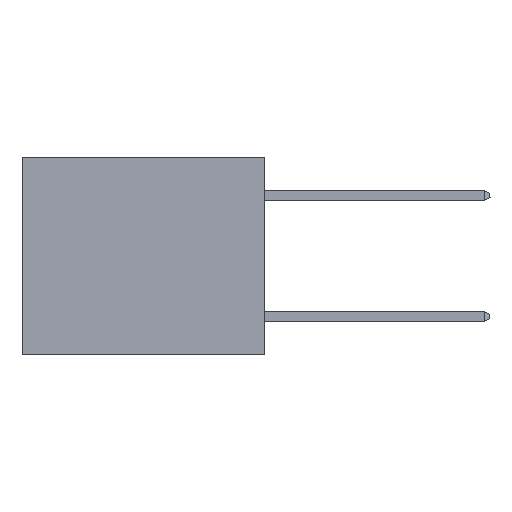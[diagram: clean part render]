
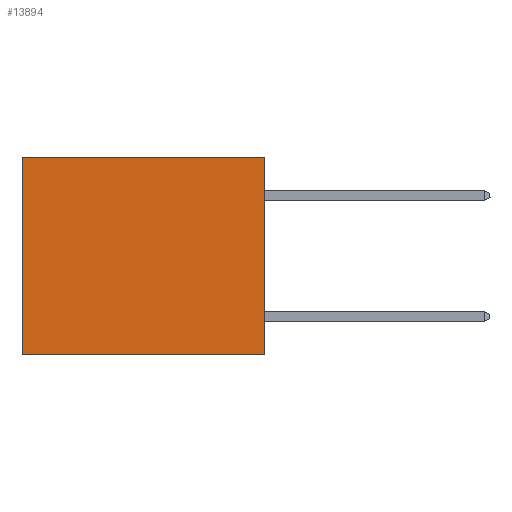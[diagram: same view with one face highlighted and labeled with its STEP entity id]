
A CAD part, left-side view. The second image highlights one B-rep face of the part: STEP entity #13894.
In plain terms, the highlighted planar face has unit normal (-1, 0, 0).
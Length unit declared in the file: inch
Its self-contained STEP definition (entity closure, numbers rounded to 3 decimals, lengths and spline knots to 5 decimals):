
#319 = EDGE_CURVE ( 'NONE', #13337, #9032, #12523, .T. ) ;
#486 = VERTEX_POINT ( 'NONE', #8522 ) ;
#912 = DIRECTION ( 'NONE',  ( 0., 1., 0. ) ) ;
#1295 = CARTESIAN_POINT ( 'NONE',  ( 0.3165, 0., -0.49 ) ) ;
#1823 = DIRECTION ( 'NONE',  ( 0., 1., 0. ) ) ;
#2435 = ORIENTED_EDGE ( 'NONE', *, *, #319, .F. ) ;
#2853 = CARTESIAN_POINT ( 'NONE',  ( 0.3165, 0., -0.49 ) ) ;
#2891 = EDGE_CURVE ( 'NONE', #486, #9357, #6642, .T. ) ;
#3004 = AXIS2_PLACEMENT_3D ( 'NONE', #20944, #11807, #22789 ) ;
#3474 = ORIENTED_EDGE ( 'NONE', *, *, #20026, .F. ) ;
#3877 = CARTESIAN_POINT ( 'NONE',  ( 0.3165, 0., -0.49 ) ) ;
#4860 = PLANE ( 'NONE',  #3004 ) ;
#5519 = DIRECTION ( 'NONE',  ( 0., 0., -1. ) ) ;
#6401 = FACE_OUTER_BOUND ( 'NONE', #19882, .T. ) ;
#6642 = LINE ( 'NONE', #7012, #15460 ) ;
#7012 = CARTESIAN_POINT ( 'NONE',  ( 0.3165, 0., 0. ) ) ;
#7449 = CARTESIAN_POINT ( 'NONE',  ( 0.3165, 0.6, -0.49 ) ) ;
#8386 = EDGE_CURVE ( 'NONE', #9357, #9032, #11478, .T. ) ;
#8522 = CARTESIAN_POINT ( 'NONE',  ( 0.3165, 0., 0. ) ) ;
#9032 = VERTEX_POINT ( 'NONE', #7449 ) ;
#9357 = VERTEX_POINT ( 'NONE', #16828 ) ;
#9439 = CARTESIAN_POINT ( 'NONE',  ( 0.3165, 0.6, -0.49 ) ) ;
#9500 = VECTOR ( 'NONE', #5519, 39.37008 ) ;
#11478 = LINE ( 'NONE', #9439, #9500 ) ;
#11807 = DIRECTION ( 'NONE',  ( 1., 0., 0. ) ) ;
#12523 = LINE ( 'NONE', #2853, #19133 ) ;
#13337 = VERTEX_POINT ( 'NONE', #3877 ) ;
#13894 = ADVANCED_FACE ( 'NONE', ( #6401 ), #4860, .F. ) ;
#14734 = LINE ( 'NONE', #1295, #22260 ) ;
#14901 = ORIENTED_EDGE ( 'NONE', *, *, #8386, .T. ) ;
#15460 = VECTOR ( 'NONE', #1823, 39.37008 ) ;
#16828 = CARTESIAN_POINT ( 'NONE',  ( 0.3165, 0.6, 0. ) ) ;
#19133 = VECTOR ( 'NONE', #912, 39.37008 ) ;
#19739 = ORIENTED_EDGE ( 'NONE', *, *, #2891, .T. ) ;
#19882 = EDGE_LOOP ( 'NONE', ( #14901, #2435, #3474, #19739 ) ) ;
#20026 = EDGE_CURVE ( 'NONE', #486, #13337, #14734, .T. ) ;
#20944 = CARTESIAN_POINT ( 'NONE',  ( 0.3165, 0., -0.49 ) ) ;
#22260 = VECTOR ( 'NONE', #23373, 39.37008 ) ;
#22789 = DIRECTION ( 'NONE',  ( 0., 0., -1. ) ) ;
#23373 = DIRECTION ( 'NONE',  ( 0., 0., -1. ) ) ;
